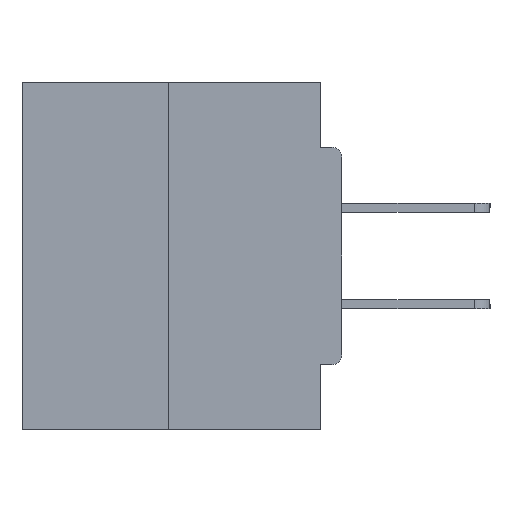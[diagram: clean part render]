
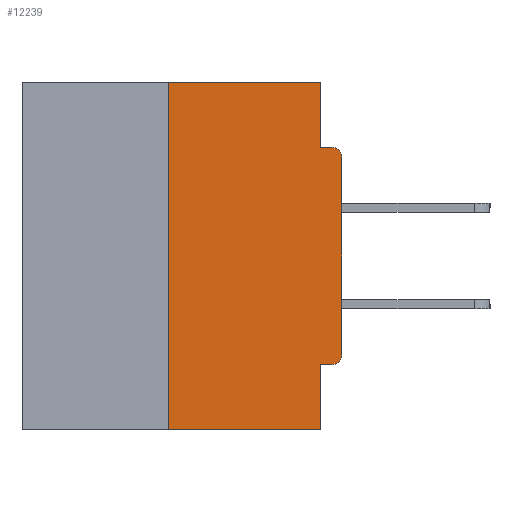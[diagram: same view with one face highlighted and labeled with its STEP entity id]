
A CAD part, left-side view. The second image highlights one B-rep face of the part: STEP entity #12239.
In plain terms, the highlighted planar face has unit normal (-1, 0, 0).
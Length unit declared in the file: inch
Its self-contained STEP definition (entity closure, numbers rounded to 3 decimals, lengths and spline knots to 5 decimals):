
#458 = DIRECTION ( 'NONE',  ( 0., 1., 0. ) ) ;
#618 = AXIS2_PLACEMENT_3D ( 'NONE', #14148, #11263, #32865 ) ;
#904 = CARTESIAN_POINT ( 'NONE',  ( 0., 0., -0.3915 ) ) ;
#1049 = LINE ( 'NONE', #29111, #11789 ) ;
#1109 = CARTESIAN_POINT ( 'NONE',  ( 0., 0.46, 0. ) ) ;
#1481 = VECTOR ( 'NONE', #24472, 39.37008 ) ;
#3794 = VERTEX_POINT ( 'NONE', #20868 ) ;
#4485 = FACE_OUTER_BOUND ( 'NONE', #21321, .T. ) ;
#5000 = EDGE_CURVE ( 'NONE', #29647, #13929, #21044, .T. ) ;
#5283 = CARTESIAN_POINT ( 'NONE',  ( 0., 0.25, -0.5 ) ) ;
#5307 = VECTOR ( 'NONE', #14140, 39.37008 ) ;
#6233 = ORIENTED_EDGE ( 'NONE', *, *, #31036, .T. ) ;
#6903 = ORIENTED_EDGE ( 'NONE', *, *, #11175, .F. ) ;
#7110 = DIRECTION ( 'NONE',  ( 0., 0., -1. ) ) ;
#7452 = CARTESIAN_POINT ( 'NONE',  ( 0., 0., -0.0935 ) ) ;
#7853 = CARTESIAN_POINT ( 'NONE',  ( 0., 0.46, -0.5 ) ) ;
#8071 = VERTEX_POINT ( 'NONE', #20764 ) ;
#8290 = ORIENTED_EDGE ( 'NONE', *, *, #33088, .F. ) ;
#8294 = LINE ( 'NONE', #7853, #31032 ) ;
#8517 = LINE ( 'NONE', #27329, #1481 ) ;
#8724 = LINE ( 'NONE', #17650, #22741 ) ;
#9137 = ORIENTED_EDGE ( 'NONE', *, *, #24459, .F. ) ;
#9276 = VERTEX_POINT ( 'NONE', #33584 ) ;
#9976 = PLANE ( 'NONE',  #20213 ) ;
#11175 = EDGE_CURVE ( 'NONE', #13929, #9276, #29845, .T. ) ;
#11263 = DIRECTION ( 'NONE',  ( -1., 0., 0. ) ) ;
#11494 = CARTESIAN_POINT ( 'NONE',  ( 0., 0.031, 0. ) ) ;
#11639 = VECTOR ( 'NONE', #27540, 39.37008 ) ;
#11713 = EDGE_CURVE ( 'NONE', #29647, #3794, #8294, .T. ) ;
#11789 = VECTOR ( 'NONE', #458, 39.37008 ) ;
#12091 = CARTESIAN_POINT ( 'NONE',  ( 0., 0.25, 0. ) ) ;
#12239 = ADVANCED_FACE ( 'NONE', ( #4485 ), #9976, .F. ) ;
#12384 = CARTESIAN_POINT ( 'NONE',  ( 0., 0.25, 0. ) ) ;
#12823 = ORIENTED_EDGE ( 'NONE', *, *, #28236, .F. ) ;
#13557 = ORIENTED_EDGE ( 'NONE', *, *, #5000, .F. ) ;
#13929 = VERTEX_POINT ( 'NONE', #12384 ) ;
#14023 = VECTOR ( 'NONE', #20061, 39.37008 ) ;
#14140 = DIRECTION ( 'NONE',  ( 0., 0., -1. ) ) ;
#14148 = CARTESIAN_POINT ( 'NONE',  ( 0., 0.015, -0.3915 ) ) ;
#15568 = DIRECTION ( 'NONE',  ( 0., -1., 0. ) ) ;
#17424 = VERTEX_POINT ( 'NONE', #28660 ) ;
#17513 = VERTEX_POINT ( 'NONE', #20827 ) ;
#17650 = CARTESIAN_POINT ( 'NONE',  ( 0., 0., 0. ) ) ;
#17711 = DIRECTION ( 'NONE',  ( 0., 0., -1. ) ) ;
#18845 = ORIENTED_EDGE ( 'NONE', *, *, #30389, .T. ) ;
#20061 = DIRECTION ( 'NONE',  ( 0., 0., 1. ) ) ;
#20213 = AXIS2_PLACEMENT_3D ( 'NONE', #25912, #28674, #17711 ) ;
#20764 = CARTESIAN_POINT ( 'NONE',  ( 0., 0.015, -0.4065 ) ) ;
#20827 = CARTESIAN_POINT ( 'NONE',  ( 0., 0.031, -0.0935 ) ) ;
#20868 = CARTESIAN_POINT ( 'NONE',  ( 0., 0.031, -0.5 ) ) ;
#21044 = LINE ( 'NONE', #12091, #14023 ) ;
#21321 = EDGE_LOOP ( 'NONE', ( #6903, #13557, #24634, #8290, #22607, #18845, #31087, #6233, #9137, #12823 ) ) ;
#21634 = AXIS2_PLACEMENT_3D ( 'NONE', #23366, #25923, #7110 ) ;
#22607 = ORIENTED_EDGE ( 'NONE', *, *, #24308, .F. ) ;
#22741 = VECTOR ( 'NONE', #33160, 39.37008 ) ;
#23366 = CARTESIAN_POINT ( 'NONE',  ( 0., 0.015, -0.1085 ) ) ;
#24019 = VERTEX_POINT ( 'NONE', #28859 ) ;
#24180 = VERTEX_POINT ( 'NONE', #29218 ) ;
#24308 = EDGE_CURVE ( 'NONE', #8071, #24180, #1049, .T. ) ;
#24459 = EDGE_CURVE ( 'NONE', #17513, #24019, #27518, .T. ) ;
#24472 = DIRECTION ( 'NONE',  ( 0., 0., -1. ) ) ;
#24634 = ORIENTED_EDGE ( 'NONE', *, *, #11713, .T. ) ;
#25912 = CARTESIAN_POINT ( 'NONE',  ( 0., 0.46, 0. ) ) ;
#25923 = DIRECTION ( 'NONE',  ( -1., 0., 0. ) ) ;
#25935 = DIRECTION ( 'NONE',  ( 0., -1., 0. ) ) ;
#27246 = EDGE_CURVE ( 'NONE', #29819, #17424, #8724, .T. ) ;
#27329 = CARTESIAN_POINT ( 'NONE',  ( 0., 0.031, -0.5 ) ) ;
#27518 = LINE ( 'NONE', #7452, #32918 ) ;
#27540 = DIRECTION ( 'NONE',  ( 0., -1., 0. ) ) ;
#28236 = EDGE_CURVE ( 'NONE', #9276, #17513, #29309, .T. ) ;
#28660 = CARTESIAN_POINT ( 'NONE',  ( 0., 0., -0.1085 ) ) ;
#28674 = DIRECTION ( 'NONE',  ( 1., 0., 0. ) ) ;
#28859 = CARTESIAN_POINT ( 'NONE',  ( 0., 0.015, -0.0935 ) ) ;
#29111 = CARTESIAN_POINT ( 'NONE',  ( 0., 0., -0.4065 ) ) ;
#29218 = CARTESIAN_POINT ( 'NONE',  ( 0., 0.031, -0.4065 ) ) ;
#29309 = LINE ( 'NONE', #11494, #5307 ) ;
#29647 = VERTEX_POINT ( 'NONE', #5283 ) ;
#29819 = VERTEX_POINT ( 'NONE', #904 ) ;
#29845 = LINE ( 'NONE', #1109, #11639 ) ;
#30154 = CIRCLE ( 'NONE', #618, 0.015 ) ;
#30389 = EDGE_CURVE ( 'NONE', #8071, #29819, #30154, .T. ) ;
#31032 = VECTOR ( 'NONE', #15568, 39.37008 ) ;
#31036 = EDGE_CURVE ( 'NONE', #17424, #24019, #31338, .T. ) ;
#31087 = ORIENTED_EDGE ( 'NONE', *, *, #27246, .T. ) ;
#31338 = CIRCLE ( 'NONE', #21634, 0.015 ) ;
#32865 = DIRECTION ( 'NONE',  ( 0., 0., -1. ) ) ;
#32918 = VECTOR ( 'NONE', #25935, 39.37008 ) ;
#33088 = EDGE_CURVE ( 'NONE', #24180, #3794, #8517, .T. ) ;
#33160 = DIRECTION ( 'NONE',  ( 0., 0., 1. ) ) ;
#33584 = CARTESIAN_POINT ( 'NONE',  ( 0., 0.031, 0. ) ) ;
